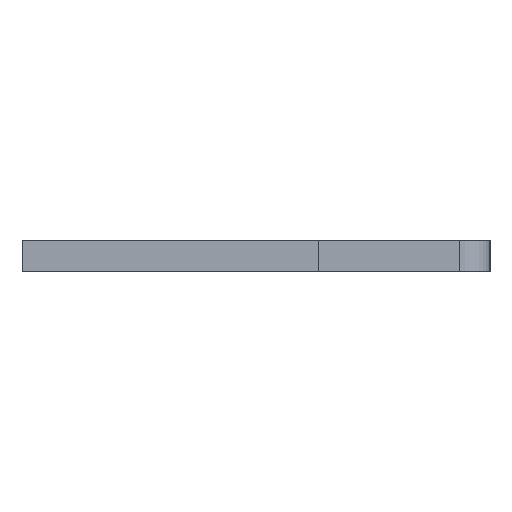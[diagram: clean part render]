
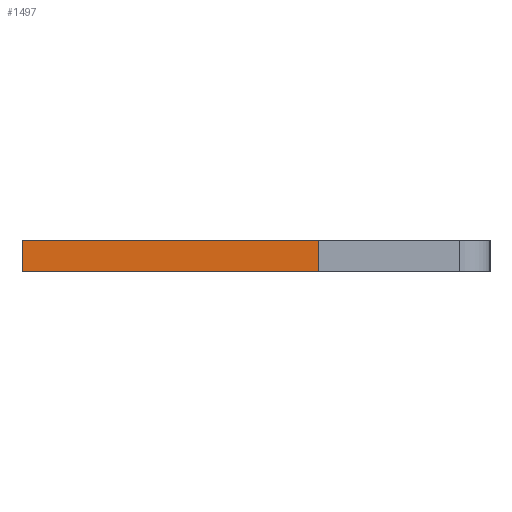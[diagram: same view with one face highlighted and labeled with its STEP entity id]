
A CAD part, left-side view. The second image highlights one B-rep face of the part: STEP entity #1497.
In plain terms, the highlighted face is planar.
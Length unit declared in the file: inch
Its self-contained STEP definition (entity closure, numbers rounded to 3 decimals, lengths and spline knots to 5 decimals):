
#26 = CARTESIAN_POINT ( 'NONE',  ( -0.01, 0.15, -0.04 ) ) ;
#67 = LINE ( 'NONE', #1405, #382 ) ;
#101 = VECTOR ( 'NONE', #536, 39.37008 ) ;
#144 = EDGE_LOOP ( 'NONE', ( #1581, #187, #484, #211 ) ) ;
#162 = LINE ( 'NONE', #1098, #101 ) ;
#164 = CARTESIAN_POINT ( 'NONE',  ( 0.01, 0.15, -0.04 ) ) ;
#187 = ORIENTED_EDGE ( 'NONE', *, *, #1316, .F. ) ;
#196 = EDGE_CURVE ( 'NONE', #628, #592, #162, .T. ) ;
#211 = ORIENTED_EDGE ( 'NONE', *, *, #196, .T. ) ;
#216 = CARTESIAN_POINT ( 'NONE',  ( 0.01, 0.15, -0.04 ) ) ;
#264 = CARTESIAN_POINT ( 'NONE',  ( -0.01, 0.15, -0.04 ) ) ;
#296 = EDGE_CURVE ( 'NONE', #592, #718, #1258, .T. ) ;
#369 = CARTESIAN_POINT ( 'NONE',  ( 0.01, 0.15, -0.04 ) ) ;
#382 = VECTOR ( 'NONE', #586, 39.37008 ) ;
#428 = VECTOR ( 'NONE', #792, 39.37008 ) ;
#441 = AXIS2_PLACEMENT_3D ( 'NONE', #216, #1175, #1307 ) ;
#484 = ORIENTED_EDGE ( 'NONE', *, *, #1012, .F. ) ;
#536 = DIRECTION ( 'NONE',  ( -1., 0., 0. ) ) ;
#555 = CARTESIAN_POINT ( 'NONE',  ( -0.01, -0.04, -0.04 ) ) ;
#586 = DIRECTION ( 'NONE',  ( 0., 1., 0. ) ) ;
#592 = VERTEX_POINT ( 'NONE', #555 ) ;
#628 = VERTEX_POINT ( 'NONE', #693 ) ;
#673 = VERTEX_POINT ( 'NONE', #164 ) ;
#693 = CARTESIAN_POINT ( 'NONE',  ( 0.01, -0.04, -0.04 ) ) ;
#718 = VERTEX_POINT ( 'NONE', #26 ) ;
#792 = DIRECTION ( 'NONE',  ( 0., 1., 0. ) ) ;
#837 = VECTOR ( 'NONE', #1431, 39.37008 ) ;
#1012 = EDGE_CURVE ( 'NONE', #628, #673, #67, .T. ) ;
#1063 = PLANE ( 'NONE',  #441 ) ;
#1098 = CARTESIAN_POINT ( 'NONE',  ( 0.01, -0.04, -0.04 ) ) ;
#1175 = DIRECTION ( 'NONE',  ( 0., 0., 1. ) ) ;
#1258 = LINE ( 'NONE', #264, #428 ) ;
#1307 = DIRECTION ( 'NONE',  ( 1., 0., 0. ) ) ;
#1316 = EDGE_CURVE ( 'NONE', #673, #718, #1661, .T. ) ;
#1405 = CARTESIAN_POINT ( 'NONE',  ( 0.01, 0.15, -0.04 ) ) ;
#1431 = DIRECTION ( 'NONE',  ( -1., 0., 0. ) ) ;
#1497 = ADVANCED_FACE ( 'NONE', ( #1498 ), #1063, .F. ) ;
#1498 = FACE_OUTER_BOUND ( 'NONE', #144, .T. ) ;
#1581 = ORIENTED_EDGE ( 'NONE', *, *, #296, .T. ) ;
#1661 = LINE ( 'NONE', #369, #837 ) ;
